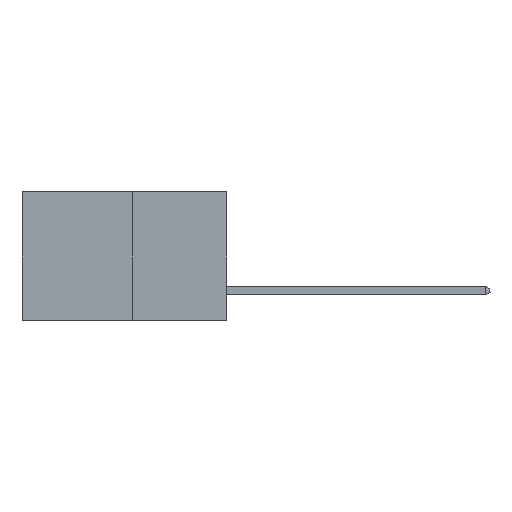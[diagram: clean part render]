
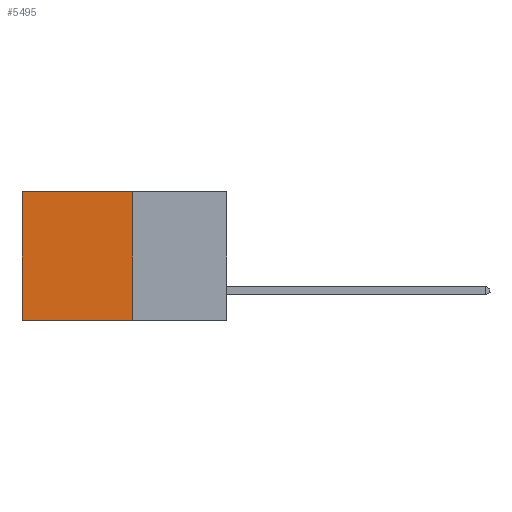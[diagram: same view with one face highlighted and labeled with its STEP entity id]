
A CAD part, left-side view. The second image highlights one B-rep face of the part: STEP entity #5495.
In plain terms, the highlighted planar face has unit normal (-1, 0, 0).
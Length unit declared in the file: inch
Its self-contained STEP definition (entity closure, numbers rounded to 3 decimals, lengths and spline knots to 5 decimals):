
#403 = ORIENTED_EDGE ( 'NONE', *, *, #5075, .F. ) ;
#1406 = VECTOR ( 'NONE', #14984, 39.37008 ) ;
#1949 = CARTESIAN_POINT ( 'NONE',  ( 0.277, 0.27, 0. ) ) ;
#1958 = VERTEX_POINT ( 'NONE', #8221 ) ;
#2139 = VECTOR ( 'NONE', #7565, 39.37008 ) ;
#2606 = AXIS2_PLACEMENT_3D ( 'NONE', #4671, #13022, #5921 ) ;
#2700 = ORIENTED_EDGE ( 'NONE', *, *, #8941, .T. ) ;
#4118 = LINE ( 'NONE', #1949, #10901 ) ;
#4671 = CARTESIAN_POINT ( 'NONE',  ( 0.277, 0.27, -0.37 ) ) ;
#4758 = LINE ( 'NONE', #7751, #7616 ) ;
#5075 = EDGE_CURVE ( 'NONE', #10552, #13789, #11795, .T. ) ;
#5177 = VERTEX_POINT ( 'NONE', #12481 ) ;
#5495 = ADVANCED_FACE ( 'NONE', ( #10611 ), #11808, .F. ) ;
#5921 = DIRECTION ( 'NONE',  ( 0., 0., -1. ) ) ;
#7208 = CARTESIAN_POINT ( 'NONE',  ( 0.277, 0.27, -0.37 ) ) ;
#7361 = EDGE_LOOP ( 'NONE', ( #2700, #403, #15517, #11527 ) ) ;
#7565 = DIRECTION ( 'NONE',  ( 0., 1., 0. ) ) ;
#7616 = VECTOR ( 'NONE', #14818, 39.37008 ) ;
#7751 = CARTESIAN_POINT ( 'NONE',  ( 0.277, 0.27, -0.37 ) ) ;
#8221 = CARTESIAN_POINT ( 'NONE',  ( 0.277, 0.59, 0. ) ) ;
#8350 = EDGE_CURVE ( 'NONE', #5177, #1958, #4118, .T. ) ;
#8941 = EDGE_CURVE ( 'NONE', #1958, #13789, #14191, .T. ) ;
#9125 = CARTESIAN_POINT ( 'NONE',  ( 0.277, 0.59, -0.37 ) ) ;
#10438 = DIRECTION ( 'NONE',  ( 0., 1., 0. ) ) ;
#10552 = VERTEX_POINT ( 'NONE', #7208 ) ;
#10611 = FACE_OUTER_BOUND ( 'NONE', #7361, .T. ) ;
#10901 = VECTOR ( 'NONE', #10438, 39.37008 ) ;
#11527 = ORIENTED_EDGE ( 'NONE', *, *, #8350, .T. ) ;
#11795 = LINE ( 'NONE', #13445, #2139 ) ;
#11808 = PLANE ( 'NONE',  #2606 ) ;
#12481 = CARTESIAN_POINT ( 'NONE',  ( 0.277, 0.27, 0. ) ) ;
#13022 = DIRECTION ( 'NONE',  ( 1., 0., 0. ) ) ;
#13065 = CARTESIAN_POINT ( 'NONE',  ( 0.277, 0.59, -0.37 ) ) ;
#13445 = CARTESIAN_POINT ( 'NONE',  ( 0.277, 0.27, -0.37 ) ) ;
#13452 = EDGE_CURVE ( 'NONE', #5177, #10552, #4758, .T. ) ;
#13789 = VERTEX_POINT ( 'NONE', #13065 ) ;
#14191 = LINE ( 'NONE', #9125, #1406 ) ;
#14818 = DIRECTION ( 'NONE',  ( 0., 0., -1. ) ) ;
#14984 = DIRECTION ( 'NONE',  ( 0., 0., -1. ) ) ;
#15517 = ORIENTED_EDGE ( 'NONE', *, *, #13452, .F. ) ;
